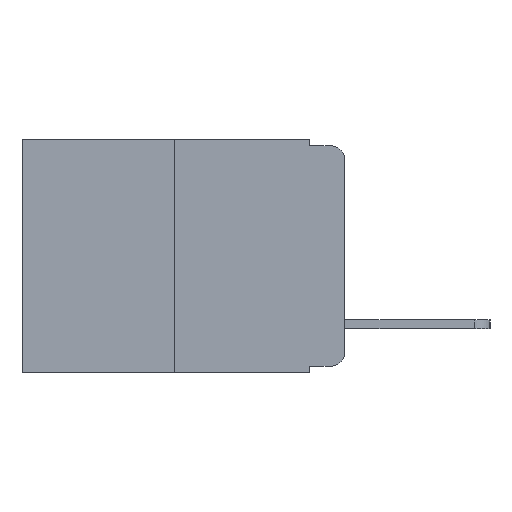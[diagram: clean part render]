
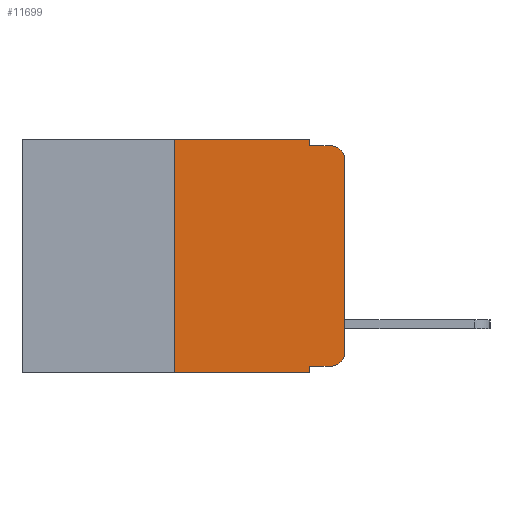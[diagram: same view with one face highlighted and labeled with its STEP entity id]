
A CAD part, left-side view. The second image highlights one B-rep face of the part: STEP entity #11699.
In plain terms, the highlighted planar face has unit normal (-1, 0, 0).
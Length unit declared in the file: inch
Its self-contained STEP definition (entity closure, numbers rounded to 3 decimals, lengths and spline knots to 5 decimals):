
#37 = VERTEX_POINT ( 'NONE', #8458 ) ;
#45 = EDGE_CURVE ( 'NONE', #2889, #4081, #11486, .T. ) ;
#193 = VERTEX_POINT ( 'NONE', #11266 ) ;
#439 = VERTEX_POINT ( 'NONE', #11034 ) ;
#573 = VECTOR ( 'NONE', #2232, 39.37008 ) ;
#648 = VECTOR ( 'NONE', #3752, 39.37008 ) ;
#714 = CARTESIAN_POINT ( 'NONE',  ( 0., 0.473, 0. ) ) ;
#930 = CARTESIAN_POINT ( 'NONE',  ( 0., 0.473, -0.343 ) ) ;
#953 = DIRECTION ( 'NONE',  ( 0., 0., -1. ) ) ;
#954 = VECTOR ( 'NONE', #10450, 39.37008 ) ;
#1195 = DIRECTION ( 'NONE',  ( 0., -1., 0. ) ) ;
#1254 = CARTESIAN_POINT ( 'NONE',  ( 0., 0., 0. ) ) ;
#1462 = VERTEX_POINT ( 'NONE', #10084 ) ;
#1767 = EDGE_CURVE ( 'NONE', #193, #37, #2926, .T. ) ;
#1931 = CARTESIAN_POINT ( 'NONE',  ( 0., 0.051, -0.333 ) ) ;
#2232 = DIRECTION ( 'NONE',  ( 0., 0., 1. ) ) ;
#2418 = AXIS2_PLACEMENT_3D ( 'NONE', #9831, #4120, #10788 ) ;
#2628 = DIRECTION ( 'NONE',  ( 0., -1., 0. ) ) ;
#2889 = VERTEX_POINT ( 'NONE', #1931 ) ;
#2926 = LINE ( 'NONE', #5231, #648 ) ;
#3059 = LINE ( 'NONE', #3199, #5352 ) ;
#3084 = EDGE_CURVE ( 'NONE', #12434, #6817, #3059, .T. ) ;
#3199 = CARTESIAN_POINT ( 'NONE',  ( 0., 0.051, -0.01 ) ) ;
#3280 = CARTESIAN_POINT ( 'NONE',  ( 0., 0.051, -0.01 ) ) ;
#3650 = VECTOR ( 'NONE', #2628, 39.37008 ) ;
#3692 = ORIENTED_EDGE ( 'NONE', *, *, #5299, .T. ) ;
#3752 = DIRECTION ( 'NONE',  ( 0., 0., 1. ) ) ;
#3797 = EDGE_CURVE ( 'NONE', #1462, #12434, #5218, .T. ) ;
#3958 = ORIENTED_EDGE ( 'NONE', *, *, #4921, .F. ) ;
#3983 = DIRECTION ( 'NONE',  ( -1., 0., 0. ) ) ;
#4081 = VERTEX_POINT ( 'NONE', #10866 ) ;
#4120 = DIRECTION ( 'NONE',  ( -1., 0., 0. ) ) ;
#4131 = ORIENTED_EDGE ( 'NONE', *, *, #45, .T. ) ;
#4542 = ORIENTED_EDGE ( 'NONE', *, *, #8166, .T. ) ;
#4921 = EDGE_CURVE ( 'NONE', #37, #1462, #8758, .T. ) ;
#5218 = LINE ( 'NONE', #9617, #7470 ) ;
#5231 = CARTESIAN_POINT ( 'NONE',  ( 0., 0.25, 0. ) ) ;
#5299 = EDGE_CURVE ( 'NONE', #439, #8378, #5740, .T. ) ;
#5352 = VECTOR ( 'NONE', #1195, 39.37008 ) ;
#5503 = CARTESIAN_POINT ( 'NONE',  ( 0., 0.051, -0.343 ) ) ;
#5631 = DIRECTION ( 'NONE',  ( 1., 0., 0. ) ) ;
#5740 = LINE ( 'NONE', #1254, #573 ) ;
#6817 = VERTEX_POINT ( 'NONE', #8651 ) ;
#7372 = LINE ( 'NONE', #930, #12101 ) ;
#7453 = ORIENTED_EDGE ( 'NONE', *, *, #3797, .F. ) ;
#7470 = VECTOR ( 'NONE', #953, 39.37008 ) ;
#7702 = CARTESIAN_POINT ( 'NONE',  ( 0., 0.051, -0.333 ) ) ;
#8079 = EDGE_CURVE ( 'NONE', #4081, #439, #11653, .T. ) ;
#8166 = EDGE_CURVE ( 'NONE', #8378, #6817, #8225, .T. ) ;
#8225 = CIRCLE ( 'NONE', #2418, 0.02 ) ;
#8378 = VERTEX_POINT ( 'NONE', #11089 ) ;
#8458 = CARTESIAN_POINT ( 'NONE',  ( 0., 0.25, 0. ) ) ;
#8638 = DIRECTION ( 'NONE',  ( 0., -1., 0. ) ) ;
#8651 = CARTESIAN_POINT ( 'NONE',  ( 0., 0.02, -0.01 ) ) ;
#8758 = LINE ( 'NONE', #714, #3650 ) ;
#9096 = EDGE_CURVE ( 'NONE', #2889, #9849, #11676, .T. ) ;
#9130 = VECTOR ( 'NONE', #10263, 39.37008 ) ;
#9201 = ORIENTED_EDGE ( 'NONE', *, *, #9096, .F. ) ;
#9288 = EDGE_CURVE ( 'NONE', #193, #9849, #7372, .T. ) ;
#9303 = CARTESIAN_POINT ( 'NONE',  ( 0., 0.051, 0. ) ) ;
#9594 = ORIENTED_EDGE ( 'NONE', *, *, #8079, .T. ) ;
#9609 = EDGE_LOOP ( 'NONE', ( #3692, #4542, #10828, #7453, #3958, #10369, #10760, #9201, #4131, #9594 ) ) ;
#9617 = CARTESIAN_POINT ( 'NONE',  ( 0., 0.051, 0. ) ) ;
#9712 = CARTESIAN_POINT ( 'NONE',  ( 0., 0.02, -0.313 ) ) ;
#9831 = CARTESIAN_POINT ( 'NONE',  ( 0., 0.02, -0.03 ) ) ;
#9849 = VERTEX_POINT ( 'NONE', #5503 ) ;
#10073 = FACE_OUTER_BOUND ( 'NONE', #9609, .T. ) ;
#10084 = CARTESIAN_POINT ( 'NONE',  ( 0., 0.051, 0. ) ) ;
#10263 = DIRECTION ( 'NONE',  ( 0., 0., -1. ) ) ;
#10369 = ORIENTED_EDGE ( 'NONE', *, *, #1767, .F. ) ;
#10450 = DIRECTION ( 'NONE',  ( 0., -1., 0. ) ) ;
#10671 = DIRECTION ( 'NONE',  ( 0., 0., -1. ) ) ;
#10760 = ORIENTED_EDGE ( 'NONE', *, *, #9288, .T. ) ;
#10788 = DIRECTION ( 'NONE',  ( 0., 0., -1. ) ) ;
#10828 = ORIENTED_EDGE ( 'NONE', *, *, #3084, .F. ) ;
#10866 = CARTESIAN_POINT ( 'NONE',  ( 0., 0.02, -0.333 ) ) ;
#11026 = AXIS2_PLACEMENT_3D ( 'NONE', #9712, #3983, #10671 ) ;
#11034 = CARTESIAN_POINT ( 'NONE',  ( 0., 0., -0.313 ) ) ;
#11089 = CARTESIAN_POINT ( 'NONE',  ( 0., 0., -0.03 ) ) ;
#11139 = PLANE ( 'NONE',  #11426 ) ;
#11266 = CARTESIAN_POINT ( 'NONE',  ( 0., 0.25, -0.343 ) ) ;
#11340 = CARTESIAN_POINT ( 'NONE',  ( 0., 0.473, 0. ) ) ;
#11426 = AXIS2_PLACEMENT_3D ( 'NONE', #11340, #5631, #12280 ) ;
#11486 = LINE ( 'NONE', #7702, #954 ) ;
#11653 = CIRCLE ( 'NONE', #11026, 0.02 ) ;
#11676 = LINE ( 'NONE', #9303, #9130 ) ;
#11699 = ADVANCED_FACE ( 'NONE', ( #10073 ), #11139, .F. ) ;
#12101 = VECTOR ( 'NONE', #8638, 39.37008 ) ;
#12280 = DIRECTION ( 'NONE',  ( 0., 0., -1. ) ) ;
#12434 = VERTEX_POINT ( 'NONE', #3280 ) ;
